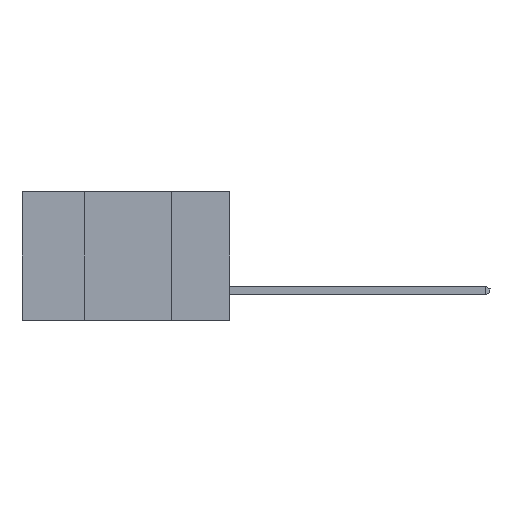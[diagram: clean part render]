
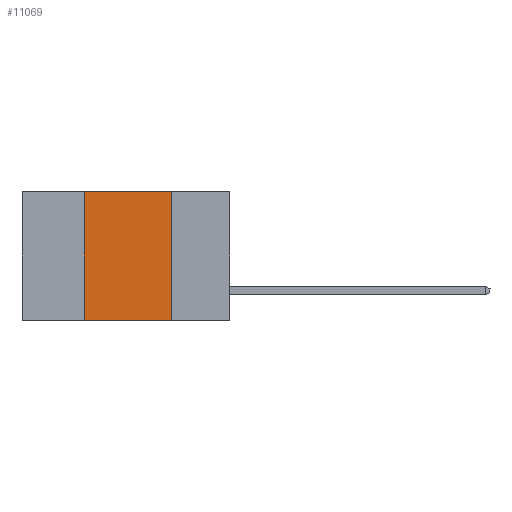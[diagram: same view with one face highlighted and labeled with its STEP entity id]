
A CAD part, left-side view. The second image highlights one B-rep face of the part: STEP entity #11069.
In plain terms, the highlighted planar face has unit normal (-1, 0, 0).
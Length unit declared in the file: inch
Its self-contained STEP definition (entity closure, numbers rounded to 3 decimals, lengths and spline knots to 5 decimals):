
#955 = LINE ( 'NONE', #11836, #17342 ) ;
#1268 = VECTOR ( 'NONE', #12602, 39.37008 ) ;
#1790 = EDGE_CURVE ( 'NONE', #11658, #12326, #15054, .T. ) ;
#1965 = DIRECTION ( 'NONE',  ( 0., -1., 0. ) ) ;
#2187 = CARTESIAN_POINT ( 'NONE',  ( 0., 0.6, 0. ) ) ;
#2656 = VERTEX_POINT ( 'NONE', #17724 ) ;
#3309 = EDGE_CURVE ( 'NONE', #11658, #12351, #955, .T. ) ;
#3788 = FACE_OUTER_BOUND ( 'NONE', #17360, .T. ) ;
#4916 = ORIENTED_EDGE ( 'NONE', *, *, #1790, .T. ) ;
#5267 = ORIENTED_EDGE ( 'NONE', *, *, #3309, .F. ) ;
#6056 = VECTOR ( 'NONE', #12587, 39.37008 ) ;
#7184 = CARTESIAN_POINT ( 'NONE',  ( 0., 0.17, -0.37 ) ) ;
#7636 = DIRECTION ( 'NONE',  ( 0., 0., 1. ) ) ;
#8548 = EDGE_CURVE ( 'NONE', #12351, #2656, #19288, .T. ) ;
#8784 = DIRECTION ( 'NONE',  ( 1., 0., 0. ) ) ;
#9181 = LINE ( 'NONE', #15675, #6056 ) ;
#9655 = ORIENTED_EDGE ( 'NONE', *, *, #11607, .F. ) ;
#10600 = CARTESIAN_POINT ( 'NONE',  ( 0., 0.42, 0. ) ) ;
#11069 = ADVANCED_FACE ( 'NONE', ( #3788 ), #13789, .F. ) ;
#11607 = EDGE_CURVE ( 'NONE', #2656, #12326, #9181, .T. ) ;
#11658 = VERTEX_POINT ( 'NONE', #14612 ) ;
#11836 = CARTESIAN_POINT ( 'NONE',  ( 0., 0.42, -0.37 ) ) ;
#12326 = VERTEX_POINT ( 'NONE', #7184 ) ;
#12351 = VERTEX_POINT ( 'NONE', #10600 ) ;
#12587 = DIRECTION ( 'NONE',  ( 0., 0., -1. ) ) ;
#12602 = DIRECTION ( 'NONE',  ( 0., -1., 0. ) ) ;
#13789 = PLANE ( 'NONE',  #14218 ) ;
#14218 = AXIS2_PLACEMENT_3D ( 'NONE', #2187, #8784, #16767 ) ;
#14572 = VECTOR ( 'NONE', #1965, 39.37008 ) ;
#14612 = CARTESIAN_POINT ( 'NONE',  ( 0., 0.42, -0.37 ) ) ;
#15054 = LINE ( 'NONE', #16546, #14572 ) ;
#15675 = CARTESIAN_POINT ( 'NONE',  ( 0., 0.17, -0.37 ) ) ;
#16546 = CARTESIAN_POINT ( 'NONE',  ( 0., 0.6, -0.37 ) ) ;
#16767 = DIRECTION ( 'NONE',  ( 0., 0., -1. ) ) ;
#17342 = VECTOR ( 'NONE', #7636, 39.37008 ) ;
#17360 = EDGE_LOOP ( 'NONE', ( #9655, #19020, #5267, #4916 ) ) ;
#17724 = CARTESIAN_POINT ( 'NONE',  ( 0., 0.17, 0. ) ) ;
#19020 = ORIENTED_EDGE ( 'NONE', *, *, #8548, .F. ) ;
#19288 = LINE ( 'NONE', #20693, #1268 ) ;
#20693 = CARTESIAN_POINT ( 'NONE',  ( 0., 0.6, 0. ) ) ;
